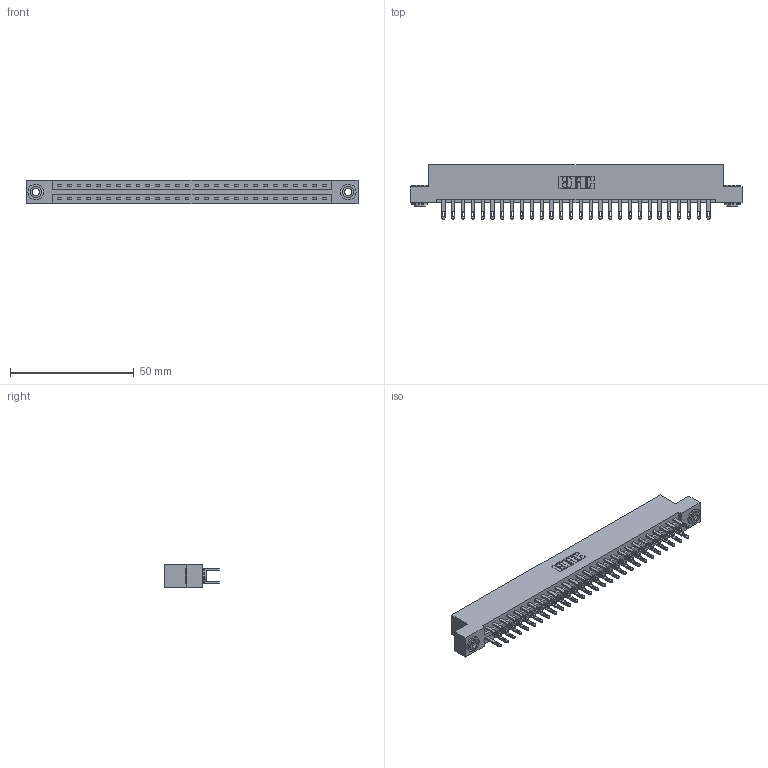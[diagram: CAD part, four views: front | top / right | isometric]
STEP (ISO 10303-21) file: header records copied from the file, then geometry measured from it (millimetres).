
FILE_DESCRIPTION (( 'STEP AP203' ), '1' );
FILE_NAME ('887-056-500-203.STEP', '2020-09-21T01:40:19', ( '' ), ( '' ), 'SwSTEP 2.0', 'SolidWorks 2020', '' );
FILE_SCHEMA (( 'CONFIG_CONTROL_DESIGN' ));
Length unit declared in the file: inch
Products named in the file (4): 345-292-001_345-293-100; 345-250-002_345-250-002-102; 837 Part_Flush Mounting Lugs - 0.156 Dia-TH; 887-056-500-203
Assembly tree (59 placements, depth 2):
  887-056-500-203
    837 Part_Flush Mounting Lugs - 0.156 Dia-TH
    345-292-001_345-293-100  x56
    345-250-002_345-250-002-102  x2
Bounding box: 133.96 x 21.85 x 9.4 mm (x, y, z)
Volume: 14121.9 mm3; surface area: 16674.6 mm2
Topology: 59 solids, 59 shells, 2952 faces, 8955 edges, 5966 vertices
Faces by surface type: plane 1872, cylinder 1072, cone 8
Entity records: 24100 total; most frequent: CARTESIAN_POINT 4045, ORIENTED_EDGE 3974, DIRECTION 3501, EDGE_CURVE 1987, VECTOR 1831, LINE 1831, VERTEX_POINT 1322, AXIS2_PLACEMENT_3D 835
